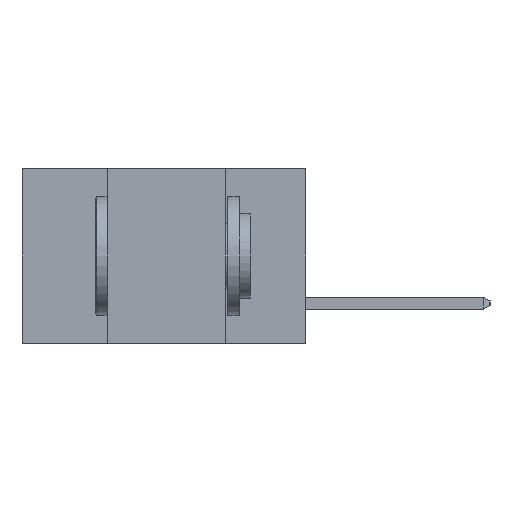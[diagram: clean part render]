
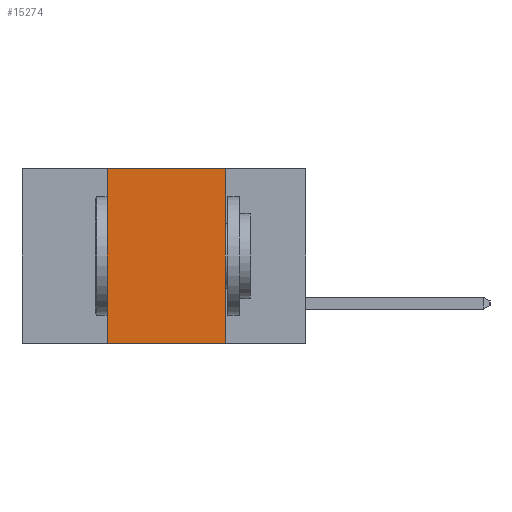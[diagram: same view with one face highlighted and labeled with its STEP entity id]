
A CAD part, left-side view. The second image highlights one B-rep face of the part: STEP entity #15274.
In plain terms, the highlighted planar face has unit normal (-1, 0, 0).
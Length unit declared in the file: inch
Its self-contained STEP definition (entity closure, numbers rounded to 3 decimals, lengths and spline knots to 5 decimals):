
#110 = AXIS2_PLACEMENT_3D ( 'NONE', #15219, #13788, #4576 ) ;
#427 = VECTOR ( 'NONE', #7305, 39.37008 ) ;
#705 = VECTOR ( 'NONE', #6427, 39.37008 ) ;
#932 = EDGE_CURVE ( 'NONE', #2588, #17187, #15232, .T. ) ;
#2588 = VERTEX_POINT ( 'NONE', #13857 ) ;
#2674 = CARTESIAN_POINT ( 'NONE',  ( 0., 0.42, 0. ) ) ;
#3050 = PLANE ( 'NONE',  #110 ) ;
#4107 = LINE ( 'NONE', #2674, #427 ) ;
#4576 = DIRECTION ( 'NONE',  ( 0., 0., -1. ) ) ;
#5120 = EDGE_LOOP ( 'NONE', ( #8435, #12804, #9192, #18150 ) ) ;
#6427 = DIRECTION ( 'NONE',  ( 0., -1., 0. ) ) ;
#6538 = CARTESIAN_POINT ( 'NONE',  ( 0., 0.6, -0.37 ) ) ;
#7305 = DIRECTION ( 'NONE',  ( 0., 0., 1. ) ) ;
#7366 = FACE_OUTER_BOUND ( 'NONE', #5120, .T. ) ;
#8434 = CARTESIAN_POINT ( 'NONE',  ( 0., 0.42, 0. ) ) ;
#8435 = ORIENTED_EDGE ( 'NONE', *, *, #932, .F. ) ;
#9192 = ORIENTED_EDGE ( 'NONE', *, *, #19663, .F. ) ;
#10387 = LINE ( 'NONE', #14100, #705 ) ;
#12011 = VERTEX_POINT ( 'NONE', #19624 ) ;
#12647 = CARTESIAN_POINT ( 'NONE',  ( 0., 0.17, -0.37 ) ) ;
#12804 = ORIENTED_EDGE ( 'NONE', *, *, #12838, .F. ) ;
#12838 = EDGE_CURVE ( 'NONE', #13044, #2588, #10387, .T. ) ;
#13044 = VERTEX_POINT ( 'NONE', #8434 ) ;
#13508 = VECTOR ( 'NONE', #17156, 39.37008 ) ;
#13788 = DIRECTION ( 'NONE',  ( 1., 0., 0. ) ) ;
#13857 = CARTESIAN_POINT ( 'NONE',  ( 0., 0.17, 0. ) ) ;
#14100 = CARTESIAN_POINT ( 'NONE',  ( 0., 0.6, 0. ) ) ;
#14387 = CARTESIAN_POINT ( 'NONE',  ( 0., 0.17, 0. ) ) ;
#15219 = CARTESIAN_POINT ( 'NONE',  ( 0., 0.6, 0. ) ) ;
#15232 = LINE ( 'NONE', #14387, #18725 ) ;
#15274 = ADVANCED_FACE ( 'NONE', ( #7366 ), #3050, .F. ) ;
#16966 = LINE ( 'NONE', #6538, #13508 ) ;
#17156 = DIRECTION ( 'NONE',  ( 0., -1., 0. ) ) ;
#17187 = VERTEX_POINT ( 'NONE', #12647 ) ;
#18150 = ORIENTED_EDGE ( 'NONE', *, *, #18690, .T. ) ;
#18690 = EDGE_CURVE ( 'NONE', #12011, #17187, #16966, .T. ) ;
#18725 = VECTOR ( 'NONE', #18862, 39.37008 ) ;
#18862 = DIRECTION ( 'NONE',  ( 0., 0., -1. ) ) ;
#19624 = CARTESIAN_POINT ( 'NONE',  ( 0., 0.42, -0.37 ) ) ;
#19663 = EDGE_CURVE ( 'NONE', #12011, #13044, #4107, .T. ) ;
